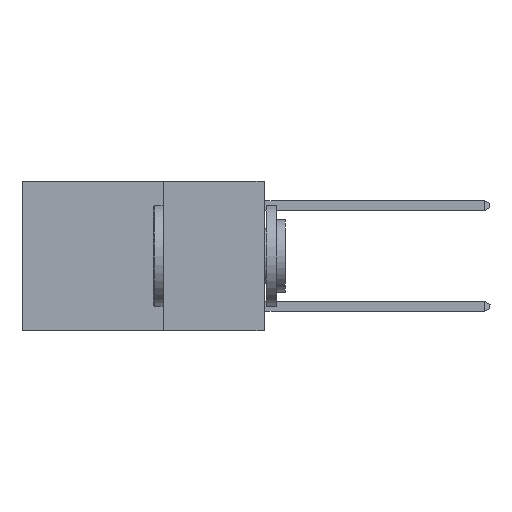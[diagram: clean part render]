
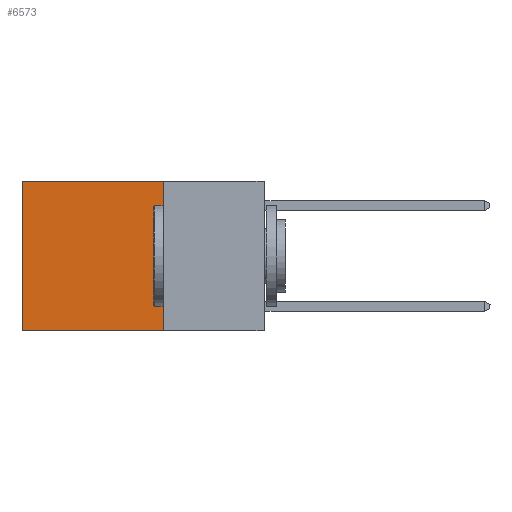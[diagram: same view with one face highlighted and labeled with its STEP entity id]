
A CAD part, left-side view. The second image highlights one B-rep face of the part: STEP entity #6573.
In plain terms, the highlighted planar face has unit normal (-1, 0, 0).
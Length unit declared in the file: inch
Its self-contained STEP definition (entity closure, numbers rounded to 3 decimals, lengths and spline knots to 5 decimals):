
#804 = PLANE ( 'NONE',  #2757 ) ;
#932 = DIRECTION ( 'NONE',  ( 0., 1., 0. ) ) ;
#939 = ORIENTED_EDGE ( 'NONE', *, *, #1707, .T. ) ;
#1318 = CARTESIAN_POINT ( 'NONE',  ( 0.2625, 0.25, 0. ) ) ;
#1465 = CARTESIAN_POINT ( 'NONE',  ( 0.2625, 0.25, 0. ) ) ;
#1475 = ORIENTED_EDGE ( 'NONE', *, *, #4173, .T. ) ;
#1617 = DIRECTION ( 'NONE',  ( 1., 0., 0. ) ) ;
#1646 = VECTOR ( 'NONE', #3627, 39.37008 ) ;
#1707 = EDGE_CURVE ( 'NONE', #2900, #1798, #1828, .T. ) ;
#1798 = VERTEX_POINT ( 'NONE', #6822 ) ;
#1828 = LINE ( 'NONE', #3594, #5661 ) ;
#2757 = AXIS2_PLACEMENT_3D ( 'NONE', #5405, #1617, #6987 ) ;
#2900 = VERTEX_POINT ( 'NONE', #4018 ) ;
#3590 = EDGE_LOOP ( 'NONE', ( #939, #5382, #4539, #1475 ) ) ;
#3594 = CARTESIAN_POINT ( 'NONE',  ( 0.2625, 0.6, 0. ) ) ;
#3627 = DIRECTION ( 'NONE',  ( 0., 0., -1. ) ) ;
#3796 = LINE ( 'NONE', #5562, #5842 ) ;
#3983 = EDGE_CURVE ( 'NONE', #9062, #8762, #9599, .T. ) ;
#4018 = CARTESIAN_POINT ( 'NONE',  ( 0.2625, 0.6, 0. ) ) ;
#4173 = EDGE_CURVE ( 'NONE', #9062, #2900, #3796, .T. ) ;
#4362 = DIRECTION ( 'NONE',  ( 0., 0., -1. ) ) ;
#4539 = ORIENTED_EDGE ( 'NONE', *, *, #3983, .F. ) ;
#5051 = FACE_OUTER_BOUND ( 'NONE', #3590, .T. ) ;
#5382 = ORIENTED_EDGE ( 'NONE', *, *, #5501, .F. ) ;
#5405 = CARTESIAN_POINT ( 'NONE',  ( 0.2625, 0.25, 0. ) ) ;
#5501 = EDGE_CURVE ( 'NONE', #8762, #1798, #6528, .T. ) ;
#5562 = CARTESIAN_POINT ( 'NONE',  ( 0.2625, 0.25, 0. ) ) ;
#5661 = VECTOR ( 'NONE', #4362, 39.37008 ) ;
#5842 = VECTOR ( 'NONE', #932, 39.37008 ) ;
#6492 = CARTESIAN_POINT ( 'NONE',  ( 0.2625, 0.25, -0.37 ) ) ;
#6528 = LINE ( 'NONE', #7207, #7831 ) ;
#6573 = ADVANCED_FACE ( 'NONE', ( #5051 ), #804, .F. ) ;
#6822 = CARTESIAN_POINT ( 'NONE',  ( 0.2625, 0.6, -0.37 ) ) ;
#6987 = DIRECTION ( 'NONE',  ( 0., 0., -1. ) ) ;
#7207 = CARTESIAN_POINT ( 'NONE',  ( 0.2625, 0.25, -0.37 ) ) ;
#7831 = VECTOR ( 'NONE', #7944, 39.37008 ) ;
#7944 = DIRECTION ( 'NONE',  ( 0., 1., 0. ) ) ;
#8762 = VERTEX_POINT ( 'NONE', #6492 ) ;
#9062 = VERTEX_POINT ( 'NONE', #1465 ) ;
#9599 = LINE ( 'NONE', #1318, #1646 ) ;
